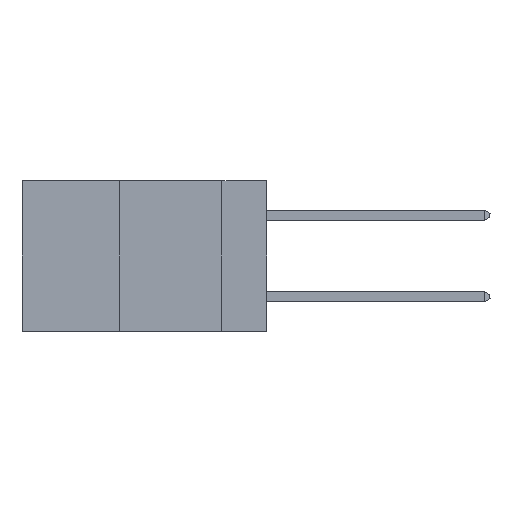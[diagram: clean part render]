
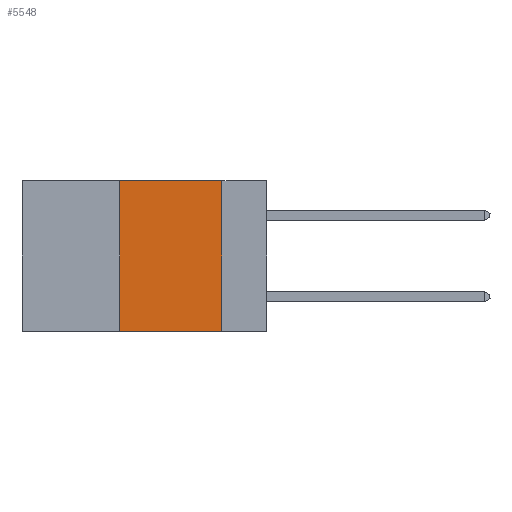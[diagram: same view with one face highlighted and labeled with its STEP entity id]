
A CAD part, left-side view. The second image highlights one B-rep face of the part: STEP entity #5548.
In plain terms, the highlighted planar face has unit normal (-1, 0, 0).
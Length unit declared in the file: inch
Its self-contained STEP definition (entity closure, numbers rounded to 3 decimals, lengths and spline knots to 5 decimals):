
#1977 = EDGE_CURVE ( 'NONE', #7398, #14223, #33687, .T. ) ;
#2672 = CARTESIAN_POINT ( 'NONE',  ( 0., 0.36, 0. ) ) ;
#2710 = CARTESIAN_POINT ( 'NONE',  ( 0., 0.6, -0.37 ) ) ;
#4560 = ORIENTED_EDGE ( 'NONE', *, *, #1977, .T. ) ;
#4679 = CARTESIAN_POINT ( 'NONE',  ( 0., 0.6, 0. ) ) ;
#5548 = ADVANCED_FACE ( 'NONE', ( #35581 ), #43342, .F. ) ;
#6245 = LINE ( 'NONE', #33024, #29436 ) ;
#7398 = VERTEX_POINT ( 'NONE', #30200 ) ;
#8272 = LINE ( 'NONE', #2672, #41673 ) ;
#9803 = CARTESIAN_POINT ( 'NONE',  ( 0., 0.11, 0. ) ) ;
#14223 = VERTEX_POINT ( 'NONE', #34224 ) ;
#14419 = VECTOR ( 'NONE', #18183, 39.37008 ) ;
#14784 = EDGE_LOOP ( 'NONE', ( #14824, #31376, #27936, #4560 ) ) ;
#14824 = ORIENTED_EDGE ( 'NONE', *, *, #41188, .F. ) ;
#15729 = CARTESIAN_POINT ( 'NONE',  ( 0., 0.36, 0. ) ) ;
#16400 = AXIS2_PLACEMENT_3D ( 'NONE', #43676, #22016, #43520 ) ;
#17379 = DIRECTION ( 'NONE',  ( 0., 0., 1. ) ) ;
#18183 = DIRECTION ( 'NONE',  ( 0., -1., 0. ) ) ;
#22016 = DIRECTION ( 'NONE',  ( 1., 0., 0. ) ) ;
#24774 = EDGE_CURVE ( 'NONE', #7398, #28693, #8272, .T. ) ;
#27908 = LINE ( 'NONE', #4679, #29573 ) ;
#27936 = ORIENTED_EDGE ( 'NONE', *, *, #24774, .F. ) ;
#28693 = VERTEX_POINT ( 'NONE', #15729 ) ;
#29436 = VECTOR ( 'NONE', #32863, 39.37008 ) ;
#29573 = VECTOR ( 'NONE', #40228, 39.37008 ) ;
#30200 = CARTESIAN_POINT ( 'NONE',  ( 0., 0.36, -0.37 ) ) ;
#31277 = VERTEX_POINT ( 'NONE', #9803 ) ;
#31376 = ORIENTED_EDGE ( 'NONE', *, *, #39777, .F. ) ;
#32863 = DIRECTION ( 'NONE',  ( 0., 0., -1. ) ) ;
#33024 = CARTESIAN_POINT ( 'NONE',  ( 0., 0.11, 0. ) ) ;
#33687 = LINE ( 'NONE', #2710, #14419 ) ;
#34224 = CARTESIAN_POINT ( 'NONE',  ( 0., 0.11, -0.37 ) ) ;
#35581 = FACE_OUTER_BOUND ( 'NONE', #14784, .T. ) ;
#39777 = EDGE_CURVE ( 'NONE', #28693, #31277, #27908, .T. ) ;
#40228 = DIRECTION ( 'NONE',  ( 0., -1., 0. ) ) ;
#41188 = EDGE_CURVE ( 'NONE', #31277, #14223, #6245, .T. ) ;
#41673 = VECTOR ( 'NONE', #17379, 39.37008 ) ;
#43342 = PLANE ( 'NONE',  #16400 ) ;
#43520 = DIRECTION ( 'NONE',  ( 0., 0., -1. ) ) ;
#43676 = CARTESIAN_POINT ( 'NONE',  ( 0., 0.6, 0. ) ) ;
